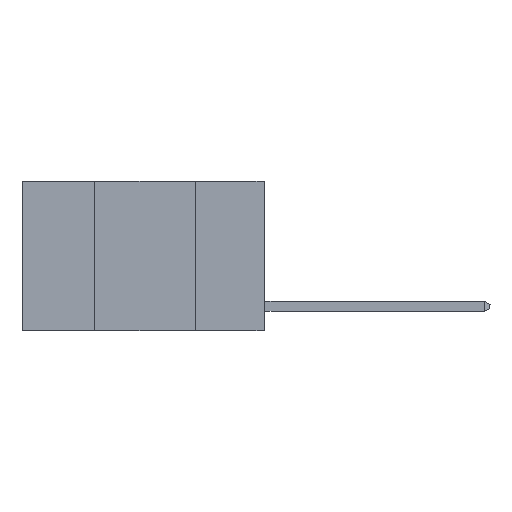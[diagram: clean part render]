
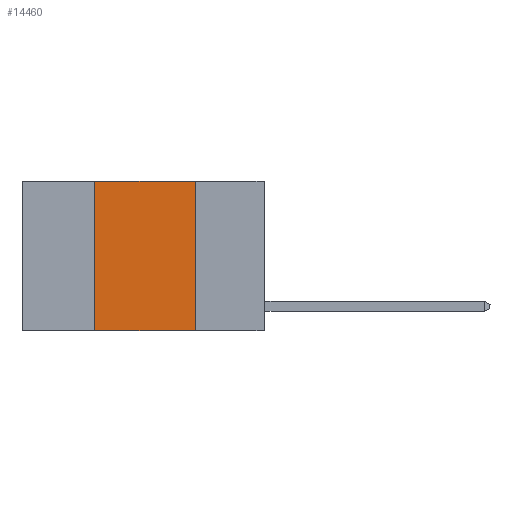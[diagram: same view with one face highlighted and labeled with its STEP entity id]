
A CAD part, left-side view. The second image highlights one B-rep face of the part: STEP entity #14460.
In plain terms, the highlighted planar face has unit normal (-1, 0, 0).
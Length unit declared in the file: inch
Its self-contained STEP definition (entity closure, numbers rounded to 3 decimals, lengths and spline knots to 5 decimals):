
#728 = EDGE_CURVE ( 'NONE', #5696, #14250, #23805, .T. ) ;
#1539 = CARTESIAN_POINT ( 'NONE',  ( 0., 0.6, -0.37 ) ) ;
#1749 = CARTESIAN_POINT ( 'NONE',  ( 0., 0.42, 0. ) ) ;
#4015 = LINE ( 'NONE', #29967, #27432 ) ;
#4951 = CARTESIAN_POINT ( 'NONE',  ( 0., 0.17, 0. ) ) ;
#5696 = VERTEX_POINT ( 'NONE', #30290 ) ;
#5901 = VECTOR ( 'NONE', #25186, 39.37008 ) ;
#8607 = VECTOR ( 'NONE', #15570, 39.37008 ) ;
#9002 = CARTESIAN_POINT ( 'NONE',  ( 0., 0.6, 0. ) ) ;
#9237 = DIRECTION ( 'NONE',  ( 0., 0., -1. ) ) ;
#9883 = ORIENTED_EDGE ( 'NONE', *, *, #19759, .F. ) ;
#10436 = VERTEX_POINT ( 'NONE', #4951 ) ;
#11318 = DIRECTION ( 'NONE',  ( 0., 0., -1. ) ) ;
#12104 = CARTESIAN_POINT ( 'NONE',  ( 0., 0.17, -0.37 ) ) ;
#12277 = EDGE_LOOP ( 'NONE', ( #29479, #9883, #23270, #14920 ) ) ;
#13088 = EDGE_CURVE ( 'NONE', #5696, #25780, #20989, .T. ) ;
#13387 = VECTOR ( 'NONE', #9237, 39.37008 ) ;
#13673 = DIRECTION ( 'NONE',  ( 0., -1., 0. ) ) ;
#14131 = LINE ( 'NONE', #20850, #13387 ) ;
#14250 = VERTEX_POINT ( 'NONE', #26860 ) ;
#14460 = ADVANCED_FACE ( 'NONE', ( #26392 ), #18247, .F. ) ;
#14920 = ORIENTED_EDGE ( 'NONE', *, *, #13088, .T. ) ;
#15570 = DIRECTION ( 'NONE',  ( 0., -1., 0. ) ) ;
#18247 = PLANE ( 'NONE',  #24442 ) ;
#19759 = EDGE_CURVE ( 'NONE', #14250, #10436, #4015, .T. ) ;
#20850 = CARTESIAN_POINT ( 'NONE',  ( 0., 0.17, 0. ) ) ;
#20989 = LINE ( 'NONE', #1539, #8607 ) ;
#23270 = ORIENTED_EDGE ( 'NONE', *, *, #728, .F. ) ;
#23805 = LINE ( 'NONE', #1749, #5901 ) ;
#23975 = EDGE_CURVE ( 'NONE', #10436, #25780, #14131, .T. ) ;
#24442 = AXIS2_PLACEMENT_3D ( 'NONE', #9002, #25311, #11318 ) ;
#25186 = DIRECTION ( 'NONE',  ( 0., 0., 1. ) ) ;
#25311 = DIRECTION ( 'NONE',  ( 1., 0., 0. ) ) ;
#25780 = VERTEX_POINT ( 'NONE', #12104 ) ;
#26392 = FACE_OUTER_BOUND ( 'NONE', #12277, .T. ) ;
#26860 = CARTESIAN_POINT ( 'NONE',  ( 0., 0.42, 0. ) ) ;
#27432 = VECTOR ( 'NONE', #13673, 39.37008 ) ;
#29479 = ORIENTED_EDGE ( 'NONE', *, *, #23975, .F. ) ;
#29967 = CARTESIAN_POINT ( 'NONE',  ( 0., 0.6, 0. ) ) ;
#30290 = CARTESIAN_POINT ( 'NONE',  ( 0., 0.42, -0.37 ) ) ;
